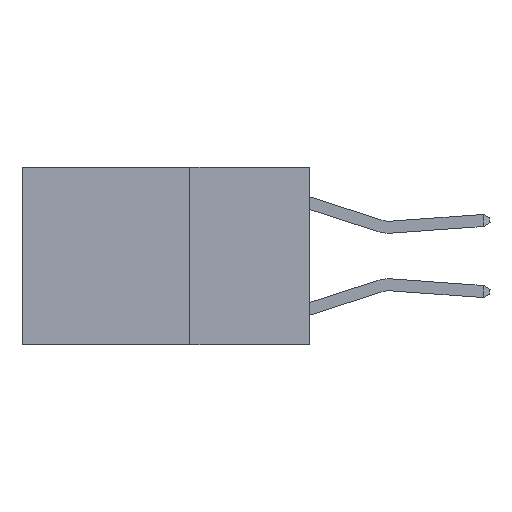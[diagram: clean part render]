
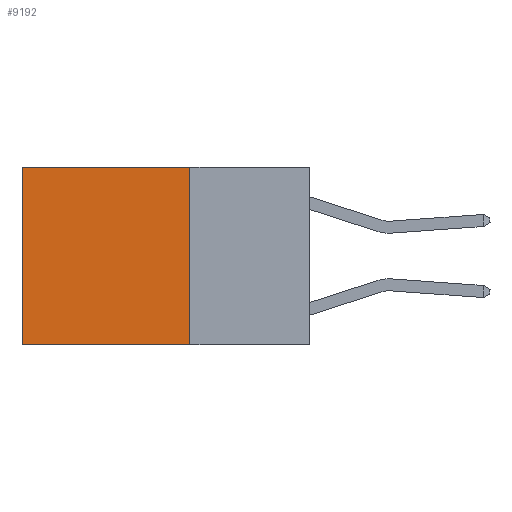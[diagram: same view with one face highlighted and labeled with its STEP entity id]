
A CAD part, left-side view. The second image highlights one B-rep face of the part: STEP entity #9192.
In plain terms, the highlighted planar face has unit normal (-1, 0, 0).
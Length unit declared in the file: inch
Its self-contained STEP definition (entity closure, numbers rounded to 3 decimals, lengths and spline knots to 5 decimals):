
#36 = DIRECTION ( 'NONE',  ( 0., 0., -1. ) ) ;
#469 = VERTEX_POINT ( 'NONE', #1493 ) ;
#923 = LINE ( 'NONE', #5900, #1280 ) ;
#1280 = VECTOR ( 'NONE', #10833, 39.37008 ) ;
#1493 = CARTESIAN_POINT ( 'NONE',  ( 0.2625, 0.6, -0.37 ) ) ;
#3365 = CARTESIAN_POINT ( 'NONE',  ( 0.2625, 0.25, -0.37 ) ) ;
#4323 = EDGE_CURVE ( 'NONE', #10243, #9234, #12175, .T. ) ;
#5301 = DIRECTION ( 'NONE',  ( 0., 1., 0. ) ) ;
#5809 = FACE_OUTER_BOUND ( 'NONE', #7832, .T. ) ;
#5900 = CARTESIAN_POINT ( 'NONE',  ( 0.2625, 0.25, -0.37 ) ) ;
#5959 = DIRECTION ( 'NONE',  ( 0., 0., -1. ) ) ;
#6082 = LINE ( 'NONE', #14790, #8391 ) ;
#7676 = EDGE_CURVE ( 'NONE', #9234, #469, #923, .T. ) ;
#7832 = EDGE_LOOP ( 'NONE', ( #14586, #11594, #13293, #9954 ) ) ;
#8045 = DIRECTION ( 'NONE',  ( 0., 0., -1. ) ) ;
#8391 = VECTOR ( 'NONE', #36, 39.37008 ) ;
#8500 = VECTOR ( 'NONE', #5959, 39.37008 ) ;
#8937 = CARTESIAN_POINT ( 'NONE',  ( 0.2625, 0.25, 0. ) ) ;
#9192 = ADVANCED_FACE ( 'NONE', ( #5809 ), #14197, .F. ) ;
#9234 = VERTEX_POINT ( 'NONE', #3365 ) ;
#9352 = AXIS2_PLACEMENT_3D ( 'NONE', #15414, #10748, #8045 ) ;
#9954 = ORIENTED_EDGE ( 'NONE', *, *, #10359, .T. ) ;
#10068 = CARTESIAN_POINT ( 'NONE',  ( 0.2625, 0.25, 0. ) ) ;
#10243 = VERTEX_POINT ( 'NONE', #10068 ) ;
#10359 = EDGE_CURVE ( 'NONE', #10243, #10593, #14094, .T. ) ;
#10593 = VERTEX_POINT ( 'NONE', #11401 ) ;
#10748 = DIRECTION ( 'NONE',  ( 1., 0., 0. ) ) ;
#10833 = DIRECTION ( 'NONE',  ( 0., 1., 0. ) ) ;
#11401 = CARTESIAN_POINT ( 'NONE',  ( 0.2625, 0.6, 0. ) ) ;
#11594 = ORIENTED_EDGE ( 'NONE', *, *, #7676, .F. ) ;
#12175 = LINE ( 'NONE', #14830, #8500 ) ;
#13293 = ORIENTED_EDGE ( 'NONE', *, *, #4323, .F. ) ;
#13830 = EDGE_CURVE ( 'NONE', #10593, #469, #6082, .T. ) ;
#14094 = LINE ( 'NONE', #8937, #15571 ) ;
#14197 = PLANE ( 'NONE',  #9352 ) ;
#14586 = ORIENTED_EDGE ( 'NONE', *, *, #13830, .T. ) ;
#14790 = CARTESIAN_POINT ( 'NONE',  ( 0.2625, 0.6, 0. ) ) ;
#14830 = CARTESIAN_POINT ( 'NONE',  ( 0.2625, 0.25, 0. ) ) ;
#15414 = CARTESIAN_POINT ( 'NONE',  ( 0.2625, 0.25, 0. ) ) ;
#15571 = VECTOR ( 'NONE', #5301, 39.37008 ) ;
